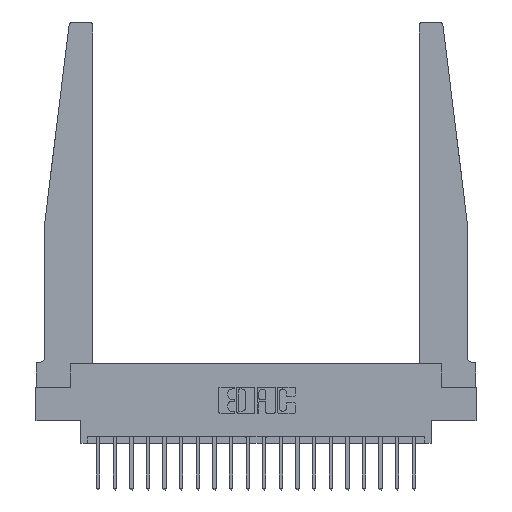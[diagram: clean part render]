
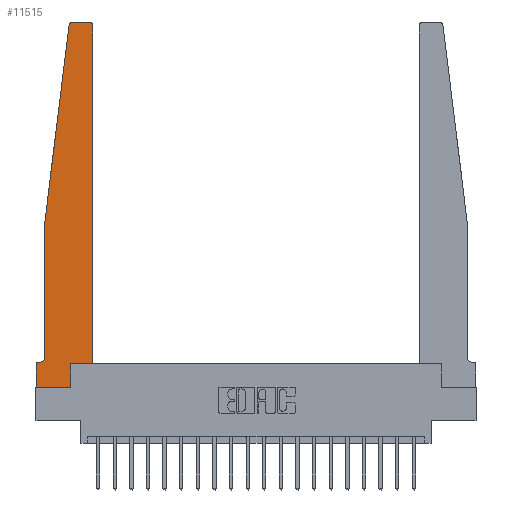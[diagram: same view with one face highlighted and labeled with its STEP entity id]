
A CAD part, top view. The second image highlights one B-rep face of the part: STEP entity #11515.
In plain terms, the highlighted planar face has unit normal (0, 0, 1).
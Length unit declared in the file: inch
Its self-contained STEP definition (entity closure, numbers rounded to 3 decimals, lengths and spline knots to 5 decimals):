
#58 = LINE ( 'NONE', #17627, #564 ) ;
#68 = VERTEX_POINT ( 'NONE', #3894 ) ;
#83 = DIRECTION ( 'NONE',  ( 0., -1., 0. ) ) ;
#92 = EDGE_CURVE ( 'NONE', #13431, #17791, #18830, .T. ) ;
#218 = EDGE_CURVE ( 'NONE', #2400, #3227, #58, .T. ) ;
#305 = DIRECTION ( 'NONE',  ( 1., 0., 0. ) ) ;
#422 = CARTESIAN_POINT ( 'NONE',  ( 0.27653, 2.72, 0.37 ) ) ;
#443 = DIRECTION ( 'NONE',  ( 0., 0., 1. ) ) ;
#521 = CARTESIAN_POINT ( 'NONE',  ( 0., 0.1875, 0.37 ) ) ;
#560 = CARTESIAN_POINT ( 'NONE',  ( 0.27653, 2.75, 0.37 ) ) ;
#564 = VECTOR ( 'NONE', #17646, 39.37008 ) ;
#786 = VECTOR ( 'NONE', #10976, 39.37008 ) ;
#1100 = VERTEX_POINT ( 'NONE', #7441 ) ;
#1125 = EDGE_CURVE ( 'NONE', #11245, #13431, #9641, .T. ) ;
#1495 = LINE ( 'NONE', #16640, #5816 ) ;
#1544 = DIRECTION ( 'NONE',  ( 1., 0., 0. ) ) ;
#1580 = VECTOR ( 'NONE', #15126, 39.37008 ) ;
#1888 = DIRECTION ( 'NONE',  ( 0., 0., -1. ) ) ;
#1918 = CIRCLE ( 'NONE', #18677, 0.05 ) ;
#2070 = EDGE_CURVE ( 'NONE', #17791, #16979, #1495, .T. ) ;
#2136 = DIRECTION ( 'NONE',  ( 1., 0., 0. ) ) ;
#2290 = CARTESIAN_POINT ( 'NONE',  ( 0.065, 0.1875, 0.37 ) ) ;
#2324 = LINE ( 'NONE', #20829, #6140 ) ;
#2400 = VERTEX_POINT ( 'NONE', #11488 ) ;
#3069 = CARTESIAN_POINT ( 'NONE',  ( 0.065, 0.2375, 0.37 ) ) ;
#3227 = VERTEX_POINT ( 'NONE', #16804 ) ;
#3649 = CARTESIAN_POINT ( 'NONE',  ( 0., 0.1875, 0.37 ) ) ;
#3822 = VERTEX_POINT ( 'NONE', #3649 ) ;
#3894 = CARTESIAN_POINT ( 'NONE',  ( 0.425, 0.18, 0.37 ) ) ;
#4149 = CARTESIAN_POINT ( 'NONE',  ( 0.25, 2.75, 0.37 ) ) ;
#4456 = DIRECTION ( 'NONE',  ( -1., 0., 0. ) ) ;
#4556 = AXIS2_PLACEMENT_3D ( 'NONE', #422, #443, #305 ) ;
#4662 = FACE_OUTER_BOUND ( 'NONE', #8170, .T. ) ;
#5282 = DIRECTION ( 'NONE',  ( -0.122, -0.992, 0. ) ) ;
#5816 = VECTOR ( 'NONE', #5282, 39.37008 ) ;
#5903 = LINE ( 'NONE', #8608, #1580 ) ;
#6017 = DIRECTION ( 'NONE',  ( 0., 0., 1. ) ) ;
#6140 = VECTOR ( 'NONE', #9498, 39.37008 ) ;
#6901 = AXIS2_PLACEMENT_3D ( 'NONE', #15718, #6017, #17379 ) ;
#7441 = CARTESIAN_POINT ( 'NONE',  ( 0.2605, 0.18, 0.37 ) ) ;
#7809 = LINE ( 'NONE', #11391, #11582 ) ;
#8170 = EDGE_LOOP ( 'NONE', ( #11885, #11426, #11968, #12265, #12506, #13156, #14748, #13243, #13724, #13269, #14001, #13936 ) ) ;
#8207 = VECTOR ( 'NONE', #15247, 39.37008 ) ;
#8316 = EDGE_CURVE ( 'NONE', #3822, #2400, #7809, .T. ) ;
#8608 = CARTESIAN_POINT ( 'NONE',  ( 0.2605, 0.18, 0.37 ) ) ;
#9398 = CIRCLE ( 'NONE', #6901, 0.03 ) ;
#9498 = DIRECTION ( 'NONE',  ( 0., -1., 0. ) ) ;
#9641 = LINE ( 'NONE', #4149, #13418 ) ;
#9814 = CARTESIAN_POINT ( 'NONE',  ( 0.065, 1.25, 0.37 ) ) ;
#10196 = PLANE ( 'NONE',  #11963 ) ;
#10976 = DIRECTION ( 'NONE',  ( 0., 1., 0. ) ) ;
#11207 = CARTESIAN_POINT ( 'NONE',  ( 0.395, 2.75, 0.37 ) ) ;
#11245 = VERTEX_POINT ( 'NONE', #11207 ) ;
#11391 = CARTESIAN_POINT ( 'NONE',  ( 0., 0., 0.37 ) ) ;
#11426 = ORIENTED_EDGE ( 'NONE', *, *, #92, .T. ) ;
#11488 = CARTESIAN_POINT ( 'NONE',  ( 0., 0., 0.37 ) ) ;
#11515 = ADVANCED_FACE ( 'NONE', ( #4662 ), #10196, .T. ) ;
#11561 = VERTEX_POINT ( 'NONE', #16811 ) ;
#11580 = CARTESIAN_POINT ( 'NONE',  ( 0.015, 0.2375, 0.37 ) ) ;
#11582 = VECTOR ( 'NONE', #83, 39.37008 ) ;
#11885 = ORIENTED_EDGE ( 'NONE', *, *, #1125, .T. ) ;
#11963 = AXIS2_PLACEMENT_3D ( 'NONE', #521, #13373, #2136 ) ;
#11968 = ORIENTED_EDGE ( 'NONE', *, *, #2070, .T. ) ;
#12171 = LINE ( 'NONE', #15783, #786 ) ;
#12265 = ORIENTED_EDGE ( 'NONE', *, *, #16143, .T. ) ;
#12506 = ORIENTED_EDGE ( 'NONE', *, *, #13312, .T. ) ;
#12527 = LINE ( 'NONE', #2290, #8207 ) ;
#13156 = ORIENTED_EDGE ( 'NONE', *, *, #19233, .T. ) ;
#13203 = DIRECTION ( 'NONE',  ( -1., 0., 0. ) ) ;
#13243 = ORIENTED_EDGE ( 'NONE', *, *, #218, .T. ) ;
#13269 = ORIENTED_EDGE ( 'NONE', *, *, #20282, .T. ) ;
#13312 = EDGE_CURVE ( 'NONE', #17574, #15818, #1918, .T. ) ;
#13373 = DIRECTION ( 'NONE',  ( 0., 0., 1. ) ) ;
#13418 = VECTOR ( 'NONE', #4456, 39.37008 ) ;
#13431 = VERTEX_POINT ( 'NONE', #560 ) ;
#13449 = CARTESIAN_POINT ( 'NONE',  ( 0.24675, 2.72367, 0.37 ) ) ;
#13724 = ORIENTED_EDGE ( 'NONE', *, *, #20541, .T. ) ;
#13936 = ORIENTED_EDGE ( 'NONE', *, *, #16733, .T. ) ;
#14001 = ORIENTED_EDGE ( 'NONE', *, *, #16770, .T. ) ;
#14748 = ORIENTED_EDGE ( 'NONE', *, *, #8316, .T. ) ;
#14768 = VECTOR ( 'NONE', #1544, 39.37008 ) ;
#15126 = DIRECTION ( 'NONE',  ( 0., 1., 0. ) ) ;
#15247 = DIRECTION ( 'NONE',  ( -1., 0., 0. ) ) ;
#15718 = CARTESIAN_POINT ( 'NONE',  ( 0.395, 2.72, 0.37 ) ) ;
#15783 = CARTESIAN_POINT ( 'NONE',  ( 0.425, 0.18, 0.37 ) ) ;
#15818 = VERTEX_POINT ( 'NONE', #20065 ) ;
#16143 = EDGE_CURVE ( 'NONE', #16979, #17574, #2324, .T. ) ;
#16640 = CARTESIAN_POINT ( 'NONE',  ( 0.065, 1.25, 0.37 ) ) ;
#16733 = EDGE_CURVE ( 'NONE', #11561, #11245, #9398, .T. ) ;
#16770 = EDGE_CURVE ( 'NONE', #68, #11561, #12171, .T. ) ;
#16804 = CARTESIAN_POINT ( 'NONE',  ( 0.2605, 0., 0.37 ) ) ;
#16811 = CARTESIAN_POINT ( 'NONE',  ( 0.425, 2.72, 0.37 ) ) ;
#16979 = VERTEX_POINT ( 'NONE', #9814 ) ;
#17379 = DIRECTION ( 'NONE',  ( 1., 0., 0. ) ) ;
#17574 = VERTEX_POINT ( 'NONE', #3069 ) ;
#17627 = CARTESIAN_POINT ( 'NONE',  ( 0., 0., 0.37 ) ) ;
#17646 = DIRECTION ( 'NONE',  ( 1., 0., 0. ) ) ;
#17791 = VERTEX_POINT ( 'NONE', #13449 ) ;
#18677 = AXIS2_PLACEMENT_3D ( 'NONE', #11580, #1888, #13203 ) ;
#18830 = CIRCLE ( 'NONE', #4556, 0.03 ) ;
#19092 = LINE ( 'NONE', #20930, #14768 ) ;
#19233 = EDGE_CURVE ( 'NONE', #15818, #3822, #12527, .T. ) ;
#20065 = CARTESIAN_POINT ( 'NONE',  ( 0.015, 0.1875, 0.37 ) ) ;
#20282 = EDGE_CURVE ( 'NONE', #1100, #68, #19092, .T. ) ;
#20541 = EDGE_CURVE ( 'NONE', #3227, #1100, #5903, .T. ) ;
#20829 = CARTESIAN_POINT ( 'NONE',  ( 0.065, 1.25, 0.37 ) ) ;
#20930 = CARTESIAN_POINT ( 'NONE',  ( 0.425, 0.18, 0.37 ) ) ;
